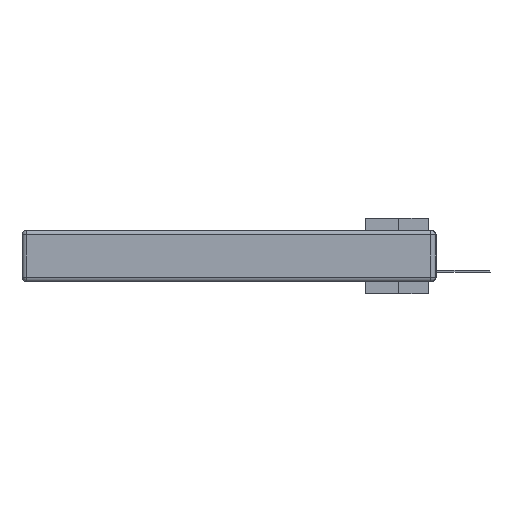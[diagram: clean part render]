
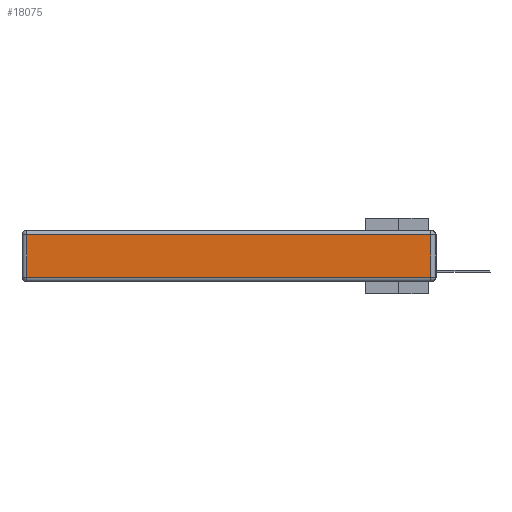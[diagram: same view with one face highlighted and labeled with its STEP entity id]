
A CAD part, left-side view. The second image highlights one B-rep face of the part: STEP entity #18075.
In plain terms, the highlighted planar face has unit normal (-1, 0, 0).
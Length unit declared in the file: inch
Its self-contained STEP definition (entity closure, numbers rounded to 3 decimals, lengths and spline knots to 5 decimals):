
#53 = CARTESIAN_POINT ( 'NONE',  ( 0., 0.03, -0.343 ) ) ;
#2801 = ORIENTED_EDGE ( 'NONE', *, *, #18213, .T. ) ;
#3028 = LINE ( 'NONE', #12783, #26313 ) ;
#3803 = DIRECTION ( 'NONE',  ( 0., 0., 1. ) ) ;
#4420 = VECTOR ( 'NONE', #21326, 39.37008 ) ;
#4815 = DIRECTION ( 'NONE',  ( 0., 0., 1. ) ) ;
#5524 = EDGE_CURVE ( 'NONE', #28316, #8676, #9239, .T. ) ;
#6066 = CARTESIAN_POINT ( 'NONE',  ( 0., 0., -0.343 ) ) ;
#6880 = ORIENTED_EDGE ( 'NONE', *, *, #5524, .T. ) ;
#7020 = EDGE_CURVE ( 'NONE', #8676, #25687, #3028, .T. ) ;
#7040 = ORIENTED_EDGE ( 'NONE', *, *, #12631, .T. ) ;
#7145 = VERTEX_POINT ( 'NONE', #22448 ) ;
#7785 = LINE ( 'NONE', #13179, #13404 ) ;
#8676 = VERTEX_POINT ( 'NONE', #28280 ) ;
#9239 = LINE ( 'NONE', #53, #29025 ) ;
#12631 = EDGE_CURVE ( 'NONE', #25687, #7145, #7785, .T. ) ;
#12783 = CARTESIAN_POINT ( 'NONE',  ( 0., 2.75, -0.03 ) ) ;
#13179 = CARTESIAN_POINT ( 'NONE',  ( 0., 2.72, -0.343 ) ) ;
#13404 = VECTOR ( 'NONE', #19821, 39.37008 ) ;
#16798 = CARTESIAN_POINT ( 'NONE',  ( 0., 0., -0.313 ) ) ;
#17495 = AXIS2_PLACEMENT_3D ( 'NONE', #6066, #26385, #3803 ) ;
#17610 = ORIENTED_EDGE ( 'NONE', *, *, #7020, .T. ) ;
#18075 = ADVANCED_FACE ( 'NONE', ( #22728 ), #19679, .T. ) ;
#18213 = EDGE_CURVE ( 'NONE', #7145, #28316, #24523, .T. ) ;
#19679 = PLANE ( 'NONE',  #17495 ) ;
#19821 = DIRECTION ( 'NONE',  ( 0., 0., -1. ) ) ;
#20030 = CARTESIAN_POINT ( 'NONE',  ( 0., 0.03, -0.313 ) ) ;
#21296 = EDGE_LOOP ( 'NONE', ( #2801, #6880, #17610, #7040 ) ) ;
#21326 = DIRECTION ( 'NONE',  ( 0., -1., 0. ) ) ;
#22448 = CARTESIAN_POINT ( 'NONE',  ( 0., 2.72, -0.313 ) ) ;
#22728 = FACE_OUTER_BOUND ( 'NONE', #21296, .T. ) ;
#24230 = DIRECTION ( 'NONE',  ( 0., 1., 0. ) ) ;
#24299 = CARTESIAN_POINT ( 'NONE',  ( 0., 2.72, -0.03 ) ) ;
#24523 = LINE ( 'NONE', #16798, #4420 ) ;
#25687 = VERTEX_POINT ( 'NONE', #24299 ) ;
#26313 = VECTOR ( 'NONE', #24230, 39.37008 ) ;
#26385 = DIRECTION ( 'NONE',  ( -1., 0., 0. ) ) ;
#28280 = CARTESIAN_POINT ( 'NONE',  ( 0., 0.03, -0.03 ) ) ;
#28316 = VERTEX_POINT ( 'NONE', #20030 ) ;
#29025 = VECTOR ( 'NONE', #4815, 39.37008 ) ;
